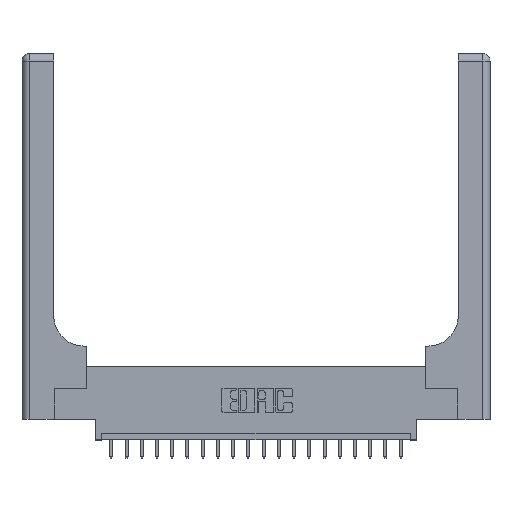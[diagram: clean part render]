
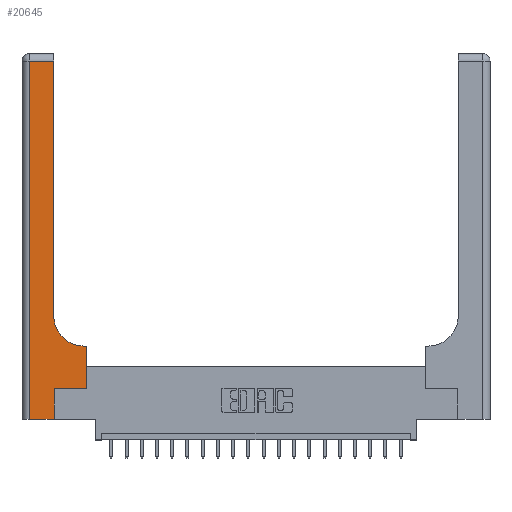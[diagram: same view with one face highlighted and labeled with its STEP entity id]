
A CAD part, top view. The second image highlights one B-rep face of the part: STEP entity #20645.
In plain terms, the highlighted planar face has unit normal (0, 0, 1).
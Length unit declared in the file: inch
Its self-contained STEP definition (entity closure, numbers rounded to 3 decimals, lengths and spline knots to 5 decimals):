
#327 = FACE_OUTER_BOUND ( 'NONE', #7286, .T. ) ;
#483 = EDGE_CURVE ( 'NONE', #15286, #8359, #16559, .T. ) ;
#797 = DIRECTION ( 'NONE',  ( 0., 0., -1. ) ) ;
#1036 = LINE ( 'NONE', #18175, #19786 ) ;
#1576 = CARTESIAN_POINT ( 'NONE',  ( 0., 2.94, 0.37 ) ) ;
#1620 = CARTESIAN_POINT ( 'NONE',  ( 0.265, 0.25, 0.37 ) ) ;
#2710 = ORIENTED_EDGE ( 'NONE', *, *, #7307, .T. ) ;
#2752 = DIRECTION ( 'NONE',  ( 0., 1., 0. ) ) ;
#2796 = CARTESIAN_POINT ( 'NONE',  ( 0.06, 2.94, 0.37 ) ) ;
#3479 = VECTOR ( 'NONE', #5795, 39.37008 ) ;
#3544 = VECTOR ( 'NONE', #13002, 39.37008 ) ;
#3775 = ORIENTED_EDGE ( 'NONE', *, *, #5610, .T. ) ;
#4158 = ORIENTED_EDGE ( 'NONE', *, *, #15631, .T. ) ;
#4362 = EDGE_CURVE ( 'NONE', #6469, #18420, #11075, .T. ) ;
#4778 = VERTEX_POINT ( 'NONE', #13582 ) ;
#4892 = DIRECTION ( 'NONE',  ( 0., -1., 0. ) ) ;
#5034 = VECTOR ( 'NONE', #5371, 39.37008 ) ;
#5119 = VECTOR ( 'NONE', #6413, 39.37008 ) ;
#5371 = DIRECTION ( 'NONE',  ( -1., 0., 0. ) ) ;
#5443 = CARTESIAN_POINT ( 'NONE',  ( 0.26, 0.6, 0.37 ) ) ;
#5610 = EDGE_CURVE ( 'NONE', #11631, #8576, #12529, .T. ) ;
#5795 = DIRECTION ( 'NONE',  ( 0., 1., 0. ) ) ;
#5963 = CARTESIAN_POINT ( 'NONE',  ( 0.528, 0.6, 0.37 ) ) ;
#5978 = ORIENTED_EDGE ( 'NONE', *, *, #7523, .T. ) ;
#6326 = ORIENTED_EDGE ( 'NONE', *, *, #4362, .T. ) ;
#6413 = DIRECTION ( 'NONE',  ( 1., 0., 0. ) ) ;
#6469 = VERTEX_POINT ( 'NONE', #19924 ) ;
#7277 = CARTESIAN_POINT ( 'NONE',  ( 0.51, 0.85, 0.37 ) ) ;
#7286 = EDGE_LOOP ( 'NONE', ( #8113, #4158, #2710, #3775, #5978, #6326, #7470, #11252, #9704 ) ) ;
#7307 = EDGE_CURVE ( 'NONE', #17825, #11631, #18532, .T. ) ;
#7470 = ORIENTED_EDGE ( 'NONE', *, *, #9289, .T. ) ;
#7523 = EDGE_CURVE ( 'NONE', #8576, #6469, #1036, .T. ) ;
#7752 = LINE ( 'NONE', #20087, #3479 ) ;
#8113 = ORIENTED_EDGE ( 'NONE', *, *, #10883, .T. ) ;
#8359 = VERTEX_POINT ( 'NONE', #17232 ) ;
#8537 = LINE ( 'NONE', #1576, #13794 ) ;
#8576 = VERTEX_POINT ( 'NONE', #19269 ) ;
#9289 = EDGE_CURVE ( 'NONE', #18420, #15286, #12361, .T. ) ;
#9704 = ORIENTED_EDGE ( 'NONE', *, *, #19681, .T. ) ;
#10259 = DIRECTION ( 'NONE',  ( 0., 1., 0. ) ) ;
#10883 = EDGE_CURVE ( 'NONE', #4778, #14575, #7752, .T. ) ;
#11075 = LINE ( 'NONE', #1620, #5119 ) ;
#11252 = ORIENTED_EDGE ( 'NONE', *, *, #483, .T. ) ;
#11631 = VERTEX_POINT ( 'NONE', #17275 ) ;
#12361 = LINE ( 'NONE', #17108, #16145 ) ;
#12529 = LINE ( 'NONE', #19203, #3544 ) ;
#12674 = PLANE ( 'NONE',  #14924 ) ;
#12704 = DIRECTION ( 'NONE',  ( -1., 0., 0. ) ) ;
#12844 = CIRCLE ( 'NONE', #14370, 0.25 ) ;
#13002 = DIRECTION ( 'NONE',  ( 1., 0., 0. ) ) ;
#13582 = CARTESIAN_POINT ( 'NONE',  ( 0.26, 0.85, 0.37 ) ) ;
#13794 = VECTOR ( 'NONE', #12704, 39.37008 ) ;
#14093 = CARTESIAN_POINT ( 'NONE',  ( 0.528, 0.25, 0.37 ) ) ;
#14252 = VECTOR ( 'NONE', #4892, 39.37008 ) ;
#14370 = AXIS2_PLACEMENT_3D ( 'NONE', #7277, #797, #15447 ) ;
#14385 = CARTESIAN_POINT ( 'NONE',  ( 0.06, 3., 0.37 ) ) ;
#14575 = VERTEX_POINT ( 'NONE', #16763 ) ;
#14924 = AXIS2_PLACEMENT_3D ( 'NONE', #17520, #17665, #19154 ) ;
#15286 = VERTEX_POINT ( 'NONE', #5963 ) ;
#15447 = DIRECTION ( 'NONE',  ( 1., 0., 0. ) ) ;
#15631 = EDGE_CURVE ( 'NONE', #14575, #17825, #8537, .T. ) ;
#16145 = VECTOR ( 'NONE', #2752, 39.37008 ) ;
#16559 = LINE ( 'NONE', #5443, #5034 ) ;
#16763 = CARTESIAN_POINT ( 'NONE',  ( 0.26, 2.94, 0.37 ) ) ;
#17108 = CARTESIAN_POINT ( 'NONE',  ( 0.528, 0.25, 0.37 ) ) ;
#17232 = CARTESIAN_POINT ( 'NONE',  ( 0.51, 0.6, 0.37 ) ) ;
#17275 = CARTESIAN_POINT ( 'NONE',  ( 0.06, 0., 0.37 ) ) ;
#17520 = CARTESIAN_POINT ( 'NONE',  ( 0., 3., 0.37 ) ) ;
#17665 = DIRECTION ( 'NONE',  ( 0., 0., -1. ) ) ;
#17825 = VERTEX_POINT ( 'NONE', #2796 ) ;
#18175 = CARTESIAN_POINT ( 'NONE',  ( 0.265, 0., 0.37 ) ) ;
#18420 = VERTEX_POINT ( 'NONE', #14093 ) ;
#18532 = LINE ( 'NONE', #14385, #14252 ) ;
#19154 = DIRECTION ( 'NONE',  ( -1., 0., 0. ) ) ;
#19203 = CARTESIAN_POINT ( 'NONE',  ( 0., 0., 0.37 ) ) ;
#19269 = CARTESIAN_POINT ( 'NONE',  ( 0.265, 0., 0.37 ) ) ;
#19681 = EDGE_CURVE ( 'NONE', #8359, #4778, #12844, .T. ) ;
#19786 = VECTOR ( 'NONE', #10259, 39.37008 ) ;
#19924 = CARTESIAN_POINT ( 'NONE',  ( 0.265, 0.25, 0.37 ) ) ;
#20087 = CARTESIAN_POINT ( 'NONE',  ( 0.26, 3., 0.37 ) ) ;
#20645 = ADVANCED_FACE ( 'NONE', ( #327 ), #12674, .F. ) ;
